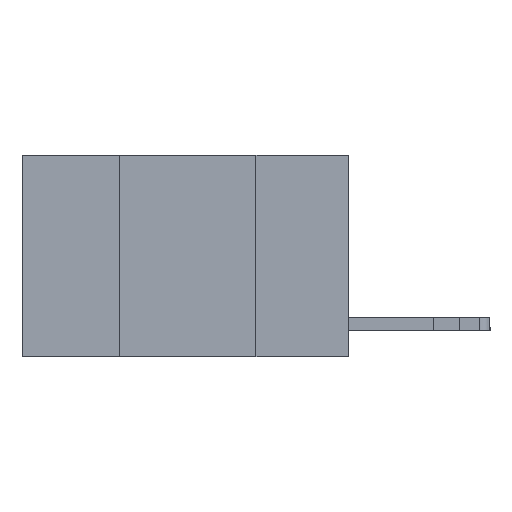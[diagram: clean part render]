
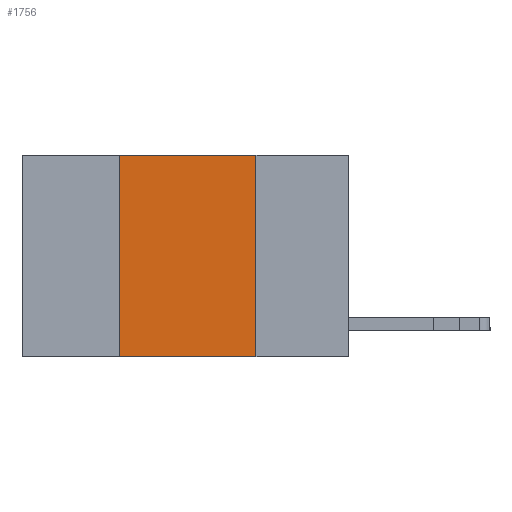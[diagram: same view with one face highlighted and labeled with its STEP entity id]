
A CAD part, left-side view. The second image highlights one B-rep face of the part: STEP entity #1756.
In plain terms, the highlighted planar face has unit normal (-1, 0, 0).
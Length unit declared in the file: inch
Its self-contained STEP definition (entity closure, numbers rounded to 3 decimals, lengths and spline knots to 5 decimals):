
#676 = LINE ( 'NONE', #2773, #3275 ) ;
#1282 = LINE ( 'NONE', #7468, #11113 ) ;
#1756 = ADVANCED_FACE ( 'NONE', ( #4972 ), #7989, .F. ) ;
#2224 = VERTEX_POINT ( 'NONE', #4891 ) ;
#2460 = VECTOR ( 'NONE', #8280, 39.37008 ) ;
#2522 = CARTESIAN_POINT ( 'NONE',  ( 0., 0.42, 0. ) ) ;
#2565 = VECTOR ( 'NONE', #4013, 39.37008 ) ;
#2773 = CARTESIAN_POINT ( 'NONE',  ( 0., 0.17, 0. ) ) ;
#3050 = VERTEX_POINT ( 'NONE', #8849 ) ;
#3261 = VERTEX_POINT ( 'NONE', #2522 ) ;
#3275 = VECTOR ( 'NONE', #11618, 39.37008 ) ;
#4013 = DIRECTION ( 'NONE',  ( 0., 0., 1. ) ) ;
#4062 = EDGE_CURVE ( 'NONE', #3050, #2224, #10333, .T. ) ;
#4891 = CARTESIAN_POINT ( 'NONE',  ( 0., 0.17, -0.37 ) ) ;
#4972 = FACE_OUTER_BOUND ( 'NONE', #7852, .T. ) ;
#5002 = LINE ( 'NONE', #12290, #2565 ) ;
#5794 = EDGE_CURVE ( 'NONE', #3050, #3261, #5002, .T. ) ;
#6265 = AXIS2_PLACEMENT_3D ( 'NONE', #7856, #12927, #10034 ) ;
#7468 = CARTESIAN_POINT ( 'NONE',  ( 0., 0.6, 0. ) ) ;
#7493 = ORIENTED_EDGE ( 'NONE', *, *, #10741, .F. ) ;
#7852 = EDGE_LOOP ( 'NONE', ( #8529, #7493, #9019, #8722 ) ) ;
#7856 = CARTESIAN_POINT ( 'NONE',  ( 0., 0.6, 0. ) ) ;
#7989 = PLANE ( 'NONE',  #6265 ) ;
#8280 = DIRECTION ( 'NONE',  ( 0., -1., 0. ) ) ;
#8529 = ORIENTED_EDGE ( 'NONE', *, *, #9712, .F. ) ;
#8722 = ORIENTED_EDGE ( 'NONE', *, *, #4062, .T. ) ;
#8849 = CARTESIAN_POINT ( 'NONE',  ( 0., 0.42, -0.37 ) ) ;
#9019 = ORIENTED_EDGE ( 'NONE', *, *, #5794, .F. ) ;
#9712 = EDGE_CURVE ( 'NONE', #10821, #2224, #676, .T. ) ;
#10034 = DIRECTION ( 'NONE',  ( 0., 0., -1. ) ) ;
#10333 = LINE ( 'NONE', #11314, #2460 ) ;
#10741 = EDGE_CURVE ( 'NONE', #3261, #10821, #1282, .T. ) ;
#10821 = VERTEX_POINT ( 'NONE', #11429 ) ;
#11113 = VECTOR ( 'NONE', #12484, 39.37008 ) ;
#11314 = CARTESIAN_POINT ( 'NONE',  ( 0., 0.6, -0.37 ) ) ;
#11429 = CARTESIAN_POINT ( 'NONE',  ( 0., 0.17, 0. ) ) ;
#11618 = DIRECTION ( 'NONE',  ( 0., 0., -1. ) ) ;
#12290 = CARTESIAN_POINT ( 'NONE',  ( 0., 0.42, 0. ) ) ;
#12484 = DIRECTION ( 'NONE',  ( 0., -1., 0. ) ) ;
#12927 = DIRECTION ( 'NONE',  ( 1., 0., 0. ) ) ;
